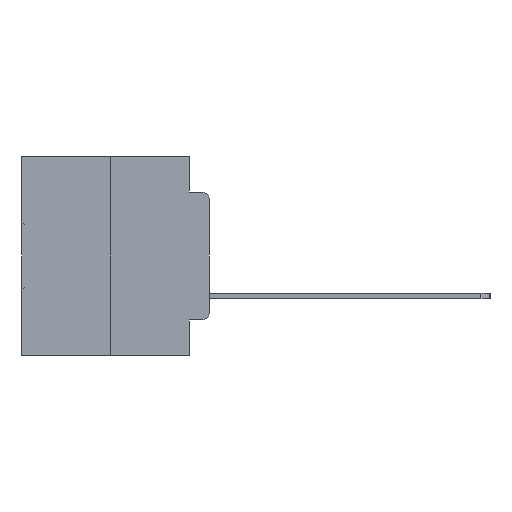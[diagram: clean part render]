
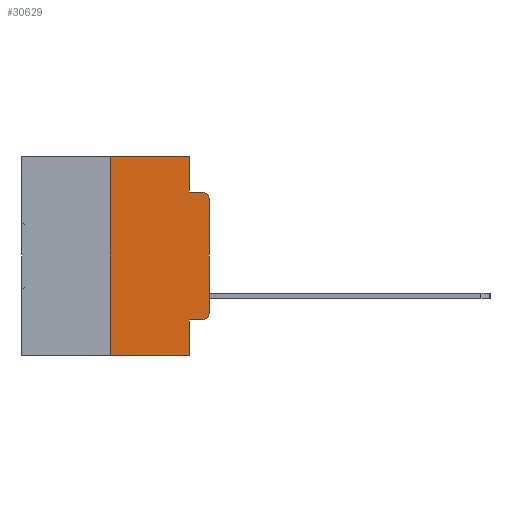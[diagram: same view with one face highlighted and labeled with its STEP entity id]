
A CAD part, left-side view. The second image highlights one B-rep face of the part: STEP entity #30629.
In plain terms, the highlighted planar face has unit normal (-1, 0, 0).
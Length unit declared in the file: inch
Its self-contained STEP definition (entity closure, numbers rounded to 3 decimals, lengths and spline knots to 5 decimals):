
#756 = VERTEX_POINT ( 'NONE', #1859 ) ;
#855 = VERTEX_POINT ( 'NONE', #20310 ) ;
#1140 = CARTESIAN_POINT ( 'NONE',  ( 0., 0.02, -0.0885 ) ) ;
#1157 = VECTOR ( 'NONE', #29256, 39.37008 ) ;
#1279 = EDGE_CURVE ( 'NONE', #14612, #855, #31905, .T. ) ;
#1296 = ORIENTED_EDGE ( 'NONE', *, *, #17261, .F. ) ;
#1556 = ORIENTED_EDGE ( 'NONE', *, *, #27564, .T. ) ;
#1567 = VERTEX_POINT ( 'NONE', #8234 ) ;
#1778 = EDGE_CURVE ( 'NONE', #27128, #1567, #17637, .T. ) ;
#1859 = CARTESIAN_POINT ( 'NONE',  ( 0., 0.25, -0.5 ) ) ;
#2180 = CARTESIAN_POINT ( 'NONE',  ( 0., 0.051, -0.5 ) ) ;
#3247 = DIRECTION ( 'NONE',  ( 1., 0., 0. ) ) ;
#3518 = CARTESIAN_POINT ( 'NONE',  ( 0., 0., -0.3915 ) ) ;
#3592 = DIRECTION ( 'NONE',  ( 0., 0., -1. ) ) ;
#4998 = CIRCLE ( 'NONE', #29280, 0.02 ) ;
#5356 = EDGE_CURVE ( 'NONE', #29093, #11716, #14756, .T. ) ;
#5860 = CARTESIAN_POINT ( 'NONE',  ( 0., 0.02, -0.3915 ) ) ;
#6294 = CIRCLE ( 'NONE', #23555, 0.02 ) ;
#6497 = AXIS2_PLACEMENT_3D ( 'NONE', #27956, #3247, #20868 ) ;
#6593 = VECTOR ( 'NONE', #3592, 39.37008 ) ;
#6843 = CARTESIAN_POINT ( 'NONE',  ( 0., 0.473, -0.5 ) ) ;
#7587 = ORIENTED_EDGE ( 'NONE', *, *, #12254, .F. ) ;
#7876 = DIRECTION ( 'NONE',  ( 0., -1., 0. ) ) ;
#8234 = CARTESIAN_POINT ( 'NONE',  ( 0., 0.051, 0. ) ) ;
#8478 = DIRECTION ( 'NONE',  ( 0., 0., -1. ) ) ;
#9940 = CARTESIAN_POINT ( 'NONE',  ( 0., 0.051, -0.4115 ) ) ;
#10770 = ORIENTED_EDGE ( 'NONE', *, *, #18113, .T. ) ;
#10889 = PLANE ( 'NONE',  #6497 ) ;
#11716 = VERTEX_POINT ( 'NONE', #2180 ) ;
#12254 = EDGE_CURVE ( 'NONE', #756, #27128, #27821, .T. ) ;
#12274 = CARTESIAN_POINT ( 'NONE',  ( 0., 0.051, 0. ) ) ;
#12486 = ORIENTED_EDGE ( 'NONE', *, *, #29132, .T. ) ;
#12944 = EDGE_LOOP ( 'NONE', ( #13316, #23606, #17059, #1296, #20502, #7587, #10770, #17602, #12486, #1556 ) ) ;
#13316 = ORIENTED_EDGE ( 'NONE', *, *, #1279, .T. ) ;
#13340 = LINE ( 'NONE', #6843, #19168 ) ;
#13971 = VERTEX_POINT ( 'NONE', #27614 ) ;
#14157 = VECTOR ( 'NONE', #24434, 39.37008 ) ;
#14612 = VERTEX_POINT ( 'NONE', #3518 ) ;
#14683 = VECTOR ( 'NONE', #7876, 39.37008 ) ;
#14746 = CARTESIAN_POINT ( 'NONE',  ( 0., 0.25, 0. ) ) ;
#14756 = LINE ( 'NONE', #12274, #1157 ) ;
#15022 = CARTESIAN_POINT ( 'NONE',  ( 0., 0.051, -0.4115 ) ) ;
#15209 = DIRECTION ( 'NONE',  ( -1., 0., 0. ) ) ;
#16315 = CARTESIAN_POINT ( 'NONE',  ( 0., 0., 0. ) ) ;
#16968 = VERTEX_POINT ( 'NONE', #22471 ) ;
#17059 = ORIENTED_EDGE ( 'NONE', *, *, #23780, .F. ) ;
#17261 = EDGE_CURVE ( 'NONE', #1567, #16968, #31181, .T. ) ;
#17602 = ORIENTED_EDGE ( 'NONE', *, *, #5356, .F. ) ;
#17637 = LINE ( 'NONE', #19809, #29649 ) ;
#18113 = EDGE_CURVE ( 'NONE', #756, #11716, #13340, .T. ) ;
#19168 = VECTOR ( 'NONE', #21777, 39.37008 ) ;
#19257 = CARTESIAN_POINT ( 'NONE',  ( 0., 0.25, 0. ) ) ;
#19809 = CARTESIAN_POINT ( 'NONE',  ( 0., 0.473, 0. ) ) ;
#20310 = CARTESIAN_POINT ( 'NONE',  ( 0., 0., -0.1085 ) ) ;
#20502 = ORIENTED_EDGE ( 'NONE', *, *, #1778, .F. ) ;
#20868 = DIRECTION ( 'NONE',  ( 0., 0., -1. ) ) ;
#20908 = DIRECTION ( 'NONE',  ( 0., -1., 0. ) ) ;
#21251 = LINE ( 'NONE', #27498, #14683 ) ;
#21565 = VECTOR ( 'NONE', #29686, 39.37008 ) ;
#21777 = DIRECTION ( 'NONE',  ( 0., -1., 0. ) ) ;
#22471 = CARTESIAN_POINT ( 'NONE',  ( 0., 0.051, -0.0885 ) ) ;
#23356 = DIRECTION ( 'NONE',  ( -1., 0., 0. ) ) ;
#23555 = AXIS2_PLACEMENT_3D ( 'NONE', #5860, #23356, #8478 ) ;
#23586 = CARTESIAN_POINT ( 'NONE',  ( 0., 0.051, 0. ) ) ;
#23606 = ORIENTED_EDGE ( 'NONE', *, *, #25379, .T. ) ;
#23780 = EDGE_CURVE ( 'NONE', #16968, #31324, #21251, .T. ) ;
#24434 = DIRECTION ( 'NONE',  ( 0., 0., 1. ) ) ;
#25379 = EDGE_CURVE ( 'NONE', #855, #31324, #4998, .T. ) ;
#25625 = VECTOR ( 'NONE', #30801, 39.37008 ) ;
#25911 = FACE_OUTER_BOUND ( 'NONE', #12944, .T. ) ;
#27128 = VERTEX_POINT ( 'NONE', #19257 ) ;
#27498 = CARTESIAN_POINT ( 'NONE',  ( 0., 0.051, -0.0885 ) ) ;
#27564 = EDGE_CURVE ( 'NONE', #13971, #14612, #6294, .T. ) ;
#27614 = CARTESIAN_POINT ( 'NONE',  ( 0., 0.02, -0.4115 ) ) ;
#27821 = LINE ( 'NONE', #14746, #14157 ) ;
#27892 = LINE ( 'NONE', #15022, #21565 ) ;
#27956 = CARTESIAN_POINT ( 'NONE',  ( 0., 0.473, 0. ) ) ;
#29093 = VERTEX_POINT ( 'NONE', #9940 ) ;
#29132 = EDGE_CURVE ( 'NONE', #29093, #13971, #27892, .T. ) ;
#29256 = DIRECTION ( 'NONE',  ( 0., 0., -1. ) ) ;
#29280 = AXIS2_PLACEMENT_3D ( 'NONE', #29652, #15209, #32023 ) ;
#29649 = VECTOR ( 'NONE', #20908, 39.37008 ) ;
#29652 = CARTESIAN_POINT ( 'NONE',  ( 0., 0.02, -0.1085 ) ) ;
#29686 = DIRECTION ( 'NONE',  ( 0., -1., 0. ) ) ;
#30629 = ADVANCED_FACE ( 'NONE', ( #25911 ), #10889, .F. ) ;
#30801 = DIRECTION ( 'NONE',  ( 0., 0., 1. ) ) ;
#31181 = LINE ( 'NONE', #23586, #6593 ) ;
#31324 = VERTEX_POINT ( 'NONE', #1140 ) ;
#31905 = LINE ( 'NONE', #16315, #25625 ) ;
#32023 = DIRECTION ( 'NONE',  ( 0., 0., -1. ) ) ;
